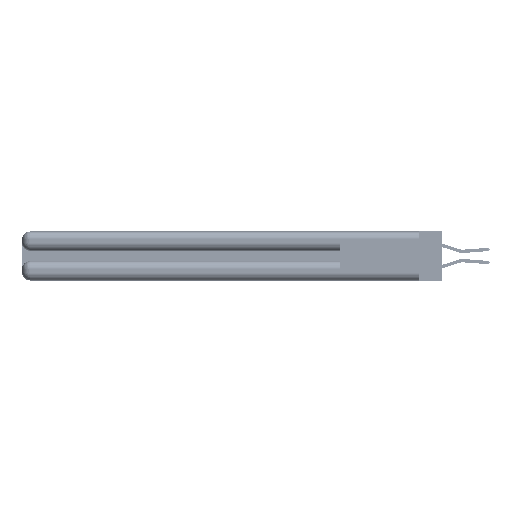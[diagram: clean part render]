
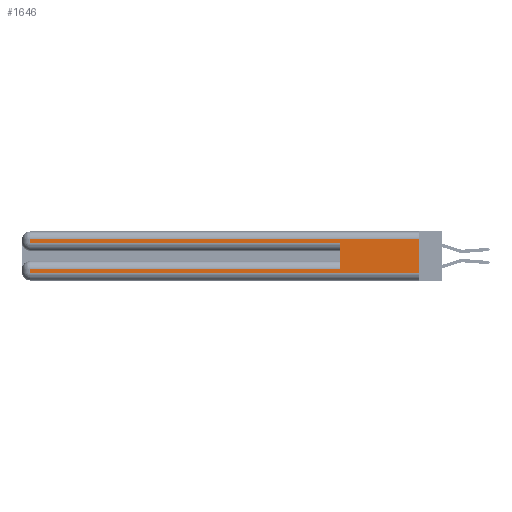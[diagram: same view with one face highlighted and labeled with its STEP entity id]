
A CAD part, left-side view. The second image highlights one B-rep face of the part: STEP entity #1646.
In plain terms, the highlighted planar face has unit normal (-1, 0, 0).
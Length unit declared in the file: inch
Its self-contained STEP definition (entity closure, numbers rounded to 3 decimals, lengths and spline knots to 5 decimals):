
#1294 = VERTEX_POINT ( 'NONE', #34868 ) ;
#1393 = DIRECTION ( 'NONE',  ( 0., -1., 0. ) ) ;
#1646 = ADVANCED_FACE ( 'NONE', ( #11657 ), #35171, .F. ) ;
#2761 = LINE ( 'NONE', #17353, #43047 ) ;
#2897 = ORIENTED_EDGE ( 'NONE', *, *, #6208, .T. ) ;
#2929 = LINE ( 'NONE', #32428, #12346 ) ;
#3528 = VERTEX_POINT ( 'NONE', #50044 ) ;
#3982 = VECTOR ( 'NONE', #19694, 39.37008 ) ;
#4617 = CARTESIAN_POINT ( 'NONE',  ( 0., 2.94, 0.31 ) ) ;
#5193 = VECTOR ( 'NONE', #51509, 39.37008 ) ;
#5253 = LINE ( 'NONE', #15686, #3982 ) ;
#6208 = EDGE_CURVE ( 'NONE', #36615, #14544, #31493, .T. ) ;
#6467 = LINE ( 'NONE', #35437, #5193 ) ;
#7206 = EDGE_CURVE ( 'NONE', #1294, #40095, #48999, .T. ) ;
#7737 = CARTESIAN_POINT ( 'NONE',  ( 0., 2.94, 0.085 ) ) ;
#8831 = EDGE_LOOP ( 'NONE', ( #29903, #45181, #2897, #33760, #16350, #44680, #43245, #42788 ) ) ;
#9526 = VECTOR ( 'NONE', #16878, 39.37008 ) ;
#11075 = CARTESIAN_POINT ( 'NONE',  ( 0., 0., 0.37 ) ) ;
#11657 = FACE_OUTER_BOUND ( 'NONE', #8831, .T. ) ;
#12346 = VECTOR ( 'NONE', #48390, 39.37008 ) ;
#14544 = VERTEX_POINT ( 'NONE', #36055 ) ;
#15088 = DIRECTION ( 'NONE',  ( 0., 0., -1. ) ) ;
#15686 = CARTESIAN_POINT ( 'NONE',  ( 0., 2.94, 0.37 ) ) ;
#16350 = ORIENTED_EDGE ( 'NONE', *, *, #19296, .F. ) ;
#16878 = DIRECTION ( 'NONE',  ( 0., 1., 0. ) ) ;
#17353 = CARTESIAN_POINT ( 'NONE',  ( 0., 0., 0.285 ) ) ;
#19010 = CARTESIAN_POINT ( 'NONE',  ( 0., 0., 0.37 ) ) ;
#19296 = EDGE_CURVE ( 'NONE', #3528, #49881, #6467, .T. ) ;
#19354 = VECTOR ( 'NONE', #31378, 39.37008 ) ;
#19694 = DIRECTION ( 'NONE',  ( 0., 0., -1. ) ) ;
#20129 = LINE ( 'NONE', #28848, #9526 ) ;
#20622 = LINE ( 'NONE', #39316, #19354 ) ;
#22290 = EDGE_CURVE ( 'NONE', #14544, #49881, #2761, .T. ) ;
#23375 = EDGE_CURVE ( 'NONE', #25359, #50384, #5253, .T. ) ;
#24282 = CARTESIAN_POINT ( 'NONE',  ( 0., 0., 0.06 ) ) ;
#25359 = VERTEX_POINT ( 'NONE', #7737 ) ;
#26025 = EDGE_CURVE ( 'NONE', #1294, #36615, #20622, .T. ) ;
#26166 = CARTESIAN_POINT ( 'NONE',  ( 0., 2.94, 0.06 ) ) ;
#28848 = CARTESIAN_POINT ( 'NONE',  ( 0., 0., 0.085 ) ) ;
#28865 = VECTOR ( 'NONE', #47157, 39.37008 ) ;
#29903 = ORIENTED_EDGE ( 'NONE', *, *, #7206, .F. ) ;
#31217 = DIRECTION ( 'NONE',  ( 0., 0., -1. ) ) ;
#31378 = DIRECTION ( 'NONE',  ( 0., 1., 0. ) ) ;
#31493 = LINE ( 'NONE', #51204, #51565 ) ;
#32428 = CARTESIAN_POINT ( 'NONE',  ( 0., 0., 0.06 ) ) ;
#33760 = ORIENTED_EDGE ( 'NONE', *, *, #22290, .T. ) ;
#33873 = EDGE_CURVE ( 'NONE', #50384, #40095, #2929, .T. ) ;
#34865 = EDGE_CURVE ( 'NONE', #3528, #25359, #20129, .T. ) ;
#34868 = CARTESIAN_POINT ( 'NONE',  ( 0., 0., 0.31 ) ) ;
#35171 = PLANE ( 'NONE',  #36256 ) ;
#35437 = CARTESIAN_POINT ( 'NONE',  ( 0., 0.6, 0.145 ) ) ;
#36055 = CARTESIAN_POINT ( 'NONE',  ( 0., 2.94, 0.285 ) ) ;
#36256 = AXIS2_PLACEMENT_3D ( 'NONE', #11075, #39205, #15088 ) ;
#36615 = VERTEX_POINT ( 'NONE', #4617 ) ;
#39084 = CARTESIAN_POINT ( 'NONE',  ( 0., 0.6, 0.285 ) ) ;
#39205 = DIRECTION ( 'NONE',  ( 1., 0., 0. ) ) ;
#39316 = CARTESIAN_POINT ( 'NONE',  ( 0., 0., 0.31 ) ) ;
#40095 = VERTEX_POINT ( 'NONE', #24282 ) ;
#42788 = ORIENTED_EDGE ( 'NONE', *, *, #33873, .T. ) ;
#43047 = VECTOR ( 'NONE', #1393, 39.37008 ) ;
#43245 = ORIENTED_EDGE ( 'NONE', *, *, #23375, .T. ) ;
#44680 = ORIENTED_EDGE ( 'NONE', *, *, #34865, .T. ) ;
#45181 = ORIENTED_EDGE ( 'NONE', *, *, #26025, .T. ) ;
#47157 = DIRECTION ( 'NONE',  ( 0., 0., -1. ) ) ;
#48390 = DIRECTION ( 'NONE',  ( 0., -1., 0. ) ) ;
#48999 = LINE ( 'NONE', #19010, #28865 ) ;
#49881 = VERTEX_POINT ( 'NONE', #39084 ) ;
#50044 = CARTESIAN_POINT ( 'NONE',  ( 0., 0.6, 0.085 ) ) ;
#50384 = VERTEX_POINT ( 'NONE', #26166 ) ;
#51204 = CARTESIAN_POINT ( 'NONE',  ( 0., 2.94, 0.37 ) ) ;
#51509 = DIRECTION ( 'NONE',  ( 0., 0., 1. ) ) ;
#51565 = VECTOR ( 'NONE', #31217, 39.37008 ) ;
